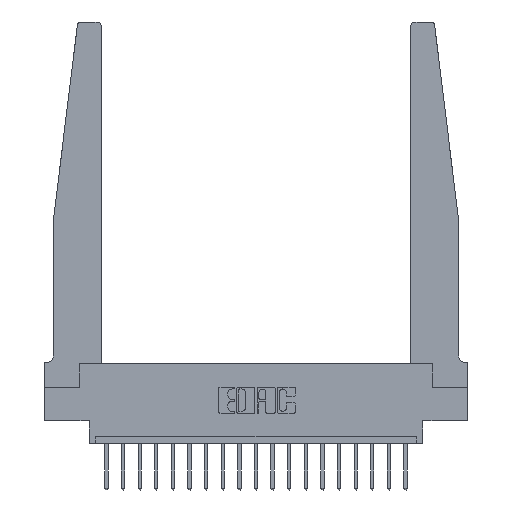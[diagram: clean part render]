
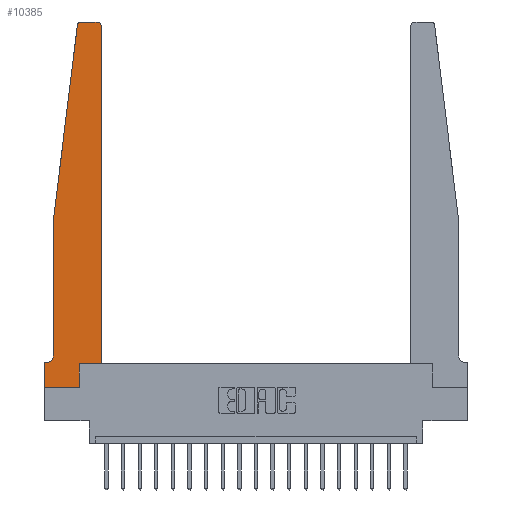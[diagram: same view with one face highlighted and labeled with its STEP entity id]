
A CAD part, top view. The second image highlights one B-rep face of the part: STEP entity #10385.
In plain terms, the highlighted planar face has unit normal (0, 0, 1).
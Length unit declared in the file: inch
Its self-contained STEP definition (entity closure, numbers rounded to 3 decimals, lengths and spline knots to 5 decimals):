
#75 = VECTOR ( 'NONE', #5653, 39.37008 ) ;
#198 = DIRECTION ( 'NONE',  ( -1., 0., 0. ) ) ;
#407 = DIRECTION ( 'NONE',  ( 0., 0., 1. ) ) ;
#475 = EDGE_CURVE ( 'NONE', #10575, #16664, #2511, .T. ) ;
#498 = CARTESIAN_POINT ( 'NONE',  ( 0.015, 0.1875, 0.37 ) ) ;
#511 = CARTESIAN_POINT ( 'NONE',  ( 0.015, 0.2375, 0.37 ) ) ;
#557 = LINE ( 'NONE', #18564, #16355 ) ;
#1070 = VECTOR ( 'NONE', #4534, 39.37008 ) ;
#1169 = VECTOR ( 'NONE', #3823, 39.37008 ) ;
#1204 = ORIENTED_EDGE ( 'NONE', *, *, #17652, .T. ) ;
#1312 = EDGE_CURVE ( 'NONE', #1962, #19079, #557, .T. ) ;
#1923 = CARTESIAN_POINT ( 'NONE',  ( 0.27653, 2.72, 0.37 ) ) ;
#1929 = DIRECTION ( 'NONE',  ( 1., 0., 0. ) ) ;
#1935 = DIRECTION ( 'NONE',  ( 0., -1., 0. ) ) ;
#1962 = VERTEX_POINT ( 'NONE', #19137 ) ;
#2296 = LINE ( 'NONE', #5534, #75 ) ;
#2359 = CARTESIAN_POINT ( 'NONE',  ( 0.2605, 0.18, 0.37 ) ) ;
#2505 = CARTESIAN_POINT ( 'NONE',  ( 0.2605, 0., 0.37 ) ) ;
#2511 = LINE ( 'NONE', #2359, #17352 ) ;
#2565 = ORIENTED_EDGE ( 'NONE', *, *, #1312, .T. ) ;
#2773 = CIRCLE ( 'NONE', #17677, 0.05 ) ;
#3128 = DIRECTION ( 'NONE',  ( -1., 0., 0. ) ) ;
#3326 = DIRECTION ( 'NONE',  ( 1., 0., 0. ) ) ;
#3448 = DIRECTION ( 'NONE',  ( 1., 0., 0. ) ) ;
#3797 = EDGE_CURVE ( 'NONE', #9218, #13601, #18199, .T. ) ;
#3823 = DIRECTION ( 'NONE',  ( -0.122, -0.992, 0. ) ) ;
#3868 = ORIENTED_EDGE ( 'NONE', *, *, #14799, .T. ) ;
#4106 = DIRECTION ( 'NONE',  ( 0., 1., 0. ) ) ;
#4301 = AXIS2_PLACEMENT_3D ( 'NONE', #18188, #19674, #18317 ) ;
#4491 = VERTEX_POINT ( 'NONE', #18640 ) ;
#4494 = VERTEX_POINT ( 'NONE', #11684 ) ;
#4534 = DIRECTION ( 'NONE',  ( 0., 1., 0. ) ) ;
#4887 = ORIENTED_EDGE ( 'NONE', *, *, #3797, .T. ) ;
#5344 = DIRECTION ( 'NONE',  ( 1., 0., 0. ) ) ;
#5446 = CARTESIAN_POINT ( 'NONE',  ( 0.2605, 0.18, 0.37 ) ) ;
#5534 = CARTESIAN_POINT ( 'NONE',  ( 0., 0., 0.37 ) ) ;
#5653 = DIRECTION ( 'NONE',  ( 0., -1., 0. ) ) ;
#5736 = ORIENTED_EDGE ( 'NONE', *, *, #19786, .T. ) ;
#5781 = VECTOR ( 'NONE', #1935, 39.37008 ) ;
#5925 = CARTESIAN_POINT ( 'NONE',  ( 0.425, 2.72, 0.37 ) ) ;
#5935 = PLANE ( 'NONE',  #4301 ) ;
#6487 = LINE ( 'NONE', #11019, #8636 ) ;
#6652 = CARTESIAN_POINT ( 'NONE',  ( 0.425, 0.18, 0.37 ) ) ;
#6758 = EDGE_CURVE ( 'NONE', #9221, #1962, #17425, .T. ) ;
#6876 = EDGE_CURVE ( 'NONE', #19079, #9218, #9036, .T. ) ;
#7661 = EDGE_CURVE ( 'NONE', #11725, #4494, #19069, .T. ) ;
#7774 = CARTESIAN_POINT ( 'NONE',  ( 0.065, 1.25, 0.37 ) ) ;
#7910 = CARTESIAN_POINT ( 'NONE',  ( 0.065, 0.1875, 0.37 ) ) ;
#8104 = DIRECTION ( 'NONE',  ( 0., 0., 1. ) ) ;
#8213 = EDGE_CURVE ( 'NONE', #15397, #9221, #12821, .T. ) ;
#8636 = VECTOR ( 'NONE', #3326, 39.37008 ) ;
#8961 = EDGE_CURVE ( 'NONE', #4494, #4491, #2296, .T. ) ;
#9036 = CIRCLE ( 'NONE', #13787, 0.03 ) ;
#9177 = VERTEX_POINT ( 'NONE', #17307 ) ;
#9218 = VERTEX_POINT ( 'NONE', #16003 ) ;
#9221 = VERTEX_POINT ( 'NONE', #5925 ) ;
#9276 = ORIENTED_EDGE ( 'NONE', *, *, #6876, .T. ) ;
#9497 = VECTOR ( 'NONE', #3128, 39.37008 ) ;
#10385 = ADVANCED_FACE ( 'NONE', ( #16348 ), #5935, .T. ) ;
#10575 = VERTEX_POINT ( 'NONE', #2505 ) ;
#11019 = CARTESIAN_POINT ( 'NONE',  ( 0.425, 0.18, 0.37 ) ) ;
#11066 = ORIENTED_EDGE ( 'NONE', *, *, #17406, .T. ) ;
#11259 = CARTESIAN_POINT ( 'NONE',  ( 0.27653, 2.75, 0.37 ) ) ;
#11368 = DIRECTION ( 'NONE',  ( 0., 0., -1. ) ) ;
#11640 = ORIENTED_EDGE ( 'NONE', *, *, #6758, .T. ) ;
#11684 = CARTESIAN_POINT ( 'NONE',  ( 0., 0.1875, 0.37 ) ) ;
#11725 = VERTEX_POINT ( 'NONE', #498 ) ;
#12123 = EDGE_LOOP ( 'NONE', ( #2565, #9276, #4887, #1204, #3868, #19003, #14227, #5736, #19746, #11066, #19707, #11640 ) ) ;
#12821 = LINE ( 'NONE', #16564, #1070 ) ;
#13244 = LINE ( 'NONE', #17317, #13473 ) ;
#13473 = VECTOR ( 'NONE', #5344, 39.37008 ) ;
#13601 = VERTEX_POINT ( 'NONE', #15291 ) ;
#13787 = AXIS2_PLACEMENT_3D ( 'NONE', #1923, #407, #3448 ) ;
#14201 = CARTESIAN_POINT ( 'NONE',  ( 0.065, 1.25, 0.37 ) ) ;
#14227 = ORIENTED_EDGE ( 'NONE', *, *, #8961, .T. ) ;
#14799 = EDGE_CURVE ( 'NONE', #9177, #11725, #2773, .T. ) ;
#15291 = CARTESIAN_POINT ( 'NONE',  ( 0.065, 1.25, 0.37 ) ) ;
#15397 = VERTEX_POINT ( 'NONE', #6652 ) ;
#16003 = CARTESIAN_POINT ( 'NONE',  ( 0.24675, 2.72367, 0.37 ) ) ;
#16348 = FACE_OUTER_BOUND ( 'NONE', #12123, .T. ) ;
#16355 = VECTOR ( 'NONE', #198, 39.37008 ) ;
#16564 = CARTESIAN_POINT ( 'NONE',  ( 0.425, 0.18, 0.37 ) ) ;
#16664 = VERTEX_POINT ( 'NONE', #5446 ) ;
#16874 = AXIS2_PLACEMENT_3D ( 'NONE', #17231, #8104, #1929 ) ;
#17231 = CARTESIAN_POINT ( 'NONE',  ( 0.395, 2.72, 0.37 ) ) ;
#17307 = CARTESIAN_POINT ( 'NONE',  ( 0.065, 0.2375, 0.37 ) ) ;
#17317 = CARTESIAN_POINT ( 'NONE',  ( 0., 0., 0.37 ) ) ;
#17352 = VECTOR ( 'NONE', #4106, 39.37008 ) ;
#17406 = EDGE_CURVE ( 'NONE', #16664, #15397, #6487, .T. ) ;
#17425 = CIRCLE ( 'NONE', #16874, 0.03 ) ;
#17652 = EDGE_CURVE ( 'NONE', #13601, #9177, #18715, .T. ) ;
#17677 = AXIS2_PLACEMENT_3D ( 'NONE', #511, #11368, #19110 ) ;
#18188 = CARTESIAN_POINT ( 'NONE',  ( 0., 0.1875, 0.37 ) ) ;
#18199 = LINE ( 'NONE', #7774, #1169 ) ;
#18317 = DIRECTION ( 'NONE',  ( 1., 0., 0. ) ) ;
#18564 = CARTESIAN_POINT ( 'NONE',  ( 0.25, 2.75, 0.37 ) ) ;
#18640 = CARTESIAN_POINT ( 'NONE',  ( 0., 0., 0.37 ) ) ;
#18715 = LINE ( 'NONE', #14201, #5781 ) ;
#19003 = ORIENTED_EDGE ( 'NONE', *, *, #7661, .T. ) ;
#19069 = LINE ( 'NONE', #7910, #9497 ) ;
#19079 = VERTEX_POINT ( 'NONE', #11259 ) ;
#19110 = DIRECTION ( 'NONE',  ( -1., 0., 0. ) ) ;
#19137 = CARTESIAN_POINT ( 'NONE',  ( 0.395, 2.75, 0.37 ) ) ;
#19674 = DIRECTION ( 'NONE',  ( 0., 0., 1. ) ) ;
#19707 = ORIENTED_EDGE ( 'NONE', *, *, #8213, .T. ) ;
#19746 = ORIENTED_EDGE ( 'NONE', *, *, #475, .T. ) ;
#19786 = EDGE_CURVE ( 'NONE', #4491, #10575, #13244, .T. ) ;
